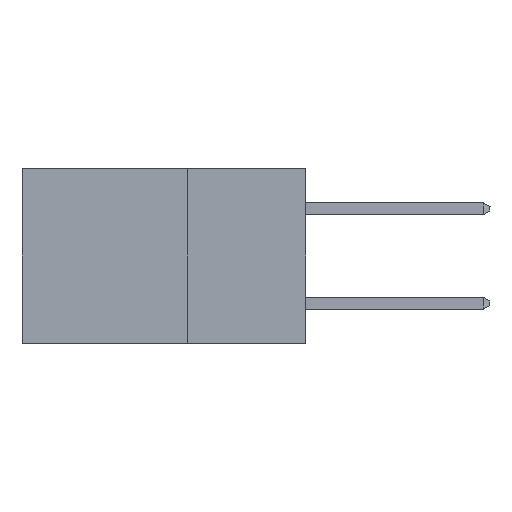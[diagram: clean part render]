
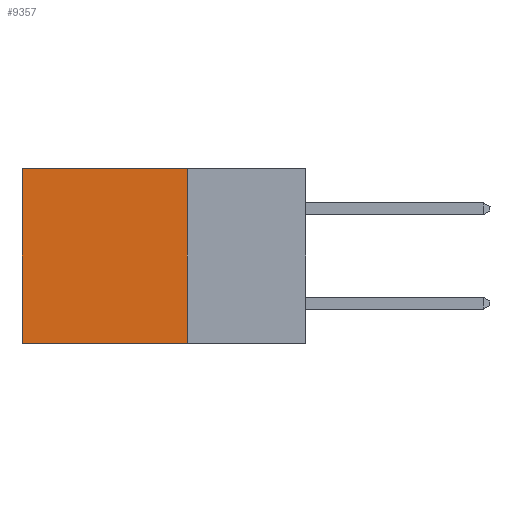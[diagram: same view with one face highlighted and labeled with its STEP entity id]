
A CAD part, left-side view. The second image highlights one B-rep face of the part: STEP entity #9357.
In plain terms, the highlighted planar face has unit normal (-1, 0, 0).
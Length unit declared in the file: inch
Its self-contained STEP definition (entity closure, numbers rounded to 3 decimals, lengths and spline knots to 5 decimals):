
#2172 = EDGE_CURVE ( 'NONE', #10660, #14827, #3769, .T. ) ;
#2179 = DIRECTION ( 'NONE',  ( 0., 1., 0. ) ) ;
#3116 = DIRECTION ( 'NONE',  ( 0., 1., 0. ) ) ;
#3321 = EDGE_LOOP ( 'NONE', ( #9916, #16668, #22585, #3974 ) ) ;
#3748 = DIRECTION ( 'NONE',  ( 1., 0., 0. ) ) ;
#3769 = LINE ( 'NONE', #27908, #21808 ) ;
#3974 = ORIENTED_EDGE ( 'NONE', *, *, #28133, .T. ) ;
#6302 = VECTOR ( 'NONE', #29187, 39.37008 ) ;
#6418 = CARTESIAN_POINT ( 'NONE',  ( 0.298, 0.6, 0. ) ) ;
#8032 = CARTESIAN_POINT ( 'NONE',  ( 0.298, 0.25, 0. ) ) ;
#9357 = ADVANCED_FACE ( 'NONE', ( #16305 ), #17340, .F. ) ;
#9434 = CARTESIAN_POINT ( 'NONE',  ( 0.298, 0.25, 0. ) ) ;
#9916 = ORIENTED_EDGE ( 'NONE', *, *, #2172, .T. ) ;
#10660 = VERTEX_POINT ( 'NONE', #6418 ) ;
#12960 = LINE ( 'NONE', #18310, #23901 ) ;
#13744 = LINE ( 'NONE', #18059, #6302 ) ;
#14827 = VERTEX_POINT ( 'NONE', #26067 ) ;
#16218 = CARTESIAN_POINT ( 'NONE',  ( 0.298, 0.25, -0.37 ) ) ;
#16305 = FACE_OUTER_BOUND ( 'NONE', #3321, .T. ) ;
#16668 = ORIENTED_EDGE ( 'NONE', *, *, #23091, .F. ) ;
#16871 = VERTEX_POINT ( 'NONE', #9434 ) ;
#17340 = PLANE ( 'NONE',  #25041 ) ;
#17415 = VERTEX_POINT ( 'NONE', #16218 ) ;
#18059 = CARTESIAN_POINT ( 'NONE',  ( 0.298, 0.25, 0. ) ) ;
#18310 = CARTESIAN_POINT ( 'NONE',  ( 0.298, 0.25, 0. ) ) ;
#20026 = LINE ( 'NONE', #23473, #22487 ) ;
#21627 = DIRECTION ( 'NONE',  ( 0., 0., -1. ) ) ;
#21808 = VECTOR ( 'NONE', #23753, 39.37008 ) ;
#22487 = VECTOR ( 'NONE', #3116, 39.37008 ) ;
#22585 = ORIENTED_EDGE ( 'NONE', *, *, #25513, .F. ) ;
#23091 = EDGE_CURVE ( 'NONE', #17415, #14827, #20026, .T. ) ;
#23473 = CARTESIAN_POINT ( 'NONE',  ( 0.298, 0.25, -0.37 ) ) ;
#23753 = DIRECTION ( 'NONE',  ( 0., 0., -1. ) ) ;
#23901 = VECTOR ( 'NONE', #2179, 39.37008 ) ;
#25041 = AXIS2_PLACEMENT_3D ( 'NONE', #8032, #3748, #21627 ) ;
#25513 = EDGE_CURVE ( 'NONE', #16871, #17415, #13744, .T. ) ;
#26067 = CARTESIAN_POINT ( 'NONE',  ( 0.298, 0.6, -0.37 ) ) ;
#27908 = CARTESIAN_POINT ( 'NONE',  ( 0.298, 0.6, 0. ) ) ;
#28133 = EDGE_CURVE ( 'NONE', #16871, #10660, #12960, .T. ) ;
#29187 = DIRECTION ( 'NONE',  ( 0., 0., -1. ) ) ;
